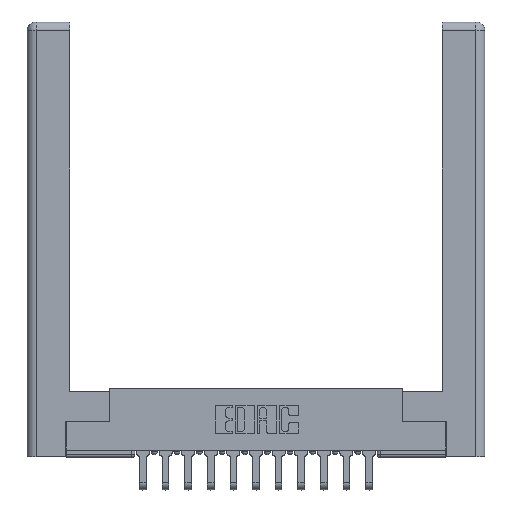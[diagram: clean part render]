
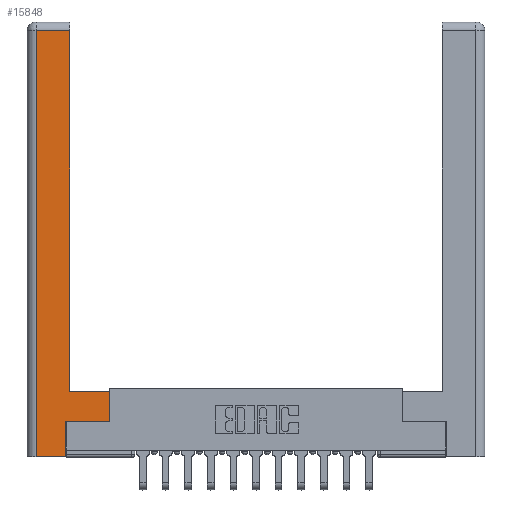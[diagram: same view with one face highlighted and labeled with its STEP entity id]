
A CAD part, top view. The second image highlights one B-rep face of the part: STEP entity #15848.
In plain terms, the highlighted planar face has unit normal (0, 0, 1).
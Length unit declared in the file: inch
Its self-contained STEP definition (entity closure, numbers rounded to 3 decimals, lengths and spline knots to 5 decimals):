
#21 = CARTESIAN_POINT ( 'NONE',  ( 0.265, 0.245, 0. ) ) ;
#48 = EDGE_CURVE ( 'NONE', #10854, #13648, #4577, .T. ) ;
#831 = VECTOR ( 'NONE', #4673, 39.37008 ) ;
#1161 = LINE ( 'NONE', #12009, #4280 ) ;
#1255 = CARTESIAN_POINT ( 'NONE',  ( 0.565, 0.45, 0. ) ) ;
#1319 = LINE ( 'NONE', #5548, #17010 ) ;
#1458 = LINE ( 'NONE', #21, #15605 ) ;
#1592 = VERTEX_POINT ( 'NONE', #5291 ) ;
#2045 = EDGE_CURVE ( 'NONE', #11021, #8924, #1319, .T. ) ;
#2308 = ORIENTED_EDGE ( 'NONE', *, *, #14729, .T. ) ;
#2418 = LINE ( 'NONE', #1255, #9904 ) ;
#2434 = LINE ( 'NONE', #6468, #12891 ) ;
#2515 = ORIENTED_EDGE ( 'NONE', *, *, #10357, .T. ) ;
#2670 = PLANE ( 'NONE',  #14595 ) ;
#2804 = EDGE_LOOP ( 'NONE', ( #8056, #16427, #3141, #2308, #14080, #10887, #13653, #2515 ) ) ;
#3123 = VECTOR ( 'NONE', #15313, 39.37008 ) ;
#3141 = ORIENTED_EDGE ( 'NONE', *, *, #11366, .T. ) ;
#3636 = CARTESIAN_POINT ( 'NONE',  ( 0.265, 0.245, 0. ) ) ;
#3809 = EDGE_CURVE ( 'NONE', #8924, #10315, #2418, .T. ) ;
#3841 = DIRECTION ( 'NONE',  ( 0., 0., -1. ) ) ;
#4144 = DIRECTION ( 'NONE',  ( 0., 1., 0. ) ) ;
#4280 = VECTOR ( 'NONE', #10565, 39.37008 ) ;
#4577 = LINE ( 'NONE', #15511, #831 ) ;
#4673 = DIRECTION ( 'NONE',  ( 0., 1., 0. ) ) ;
#4725 = EDGE_CURVE ( 'NONE', #11416, #11021, #1458, .T. ) ;
#5261 = CARTESIAN_POINT ( 'NONE',  ( 0.0615, 2.94, 0. ) ) ;
#5291 = CARTESIAN_POINT ( 'NONE',  ( 0.0615, 2.94, 0. ) ) ;
#5367 = VERTEX_POINT ( 'NONE', #11301 ) ;
#5545 = CARTESIAN_POINT ( 'NONE',  ( 0.565, 0.245, 0. ) ) ;
#5548 = CARTESIAN_POINT ( 'NONE',  ( 0.565, 0.245, 0. ) ) ;
#6095 = CARTESIAN_POINT ( 'NONE',  ( 0.565, 0.45, 0. ) ) ;
#6468 = CARTESIAN_POINT ( 'NONE',  ( 0.0615, 0., 0. ) ) ;
#6781 = DIRECTION ( 'NONE',  ( -1., 0., 0. ) ) ;
#8056 = ORIENTED_EDGE ( 'NONE', *, *, #48, .T. ) ;
#8129 = LINE ( 'NONE', #5261, #11469 ) ;
#8924 = VERTEX_POINT ( 'NONE', #5545 ) ;
#9904 = VECTOR ( 'NONE', #16128, 39.37008 ) ;
#10315 = VERTEX_POINT ( 'NONE', #6095 ) ;
#10357 = EDGE_CURVE ( 'NONE', #10315, #10854, #12900, .T. ) ;
#10565 = DIRECTION ( 'NONE',  ( 1., 0., 0. ) ) ;
#10774 = CARTESIAN_POINT ( 'NONE',  ( 0.265, 0., 0. ) ) ;
#10854 = VERTEX_POINT ( 'NONE', #16833 ) ;
#10887 = ORIENTED_EDGE ( 'NONE', *, *, #2045, .T. ) ;
#11021 = VERTEX_POINT ( 'NONE', #3636 ) ;
#11117 = EDGE_CURVE ( 'NONE', #13648, #1592, #8129, .T. ) ;
#11301 = CARTESIAN_POINT ( 'NONE',  ( 0.0615, 0., 0. ) ) ;
#11366 = EDGE_CURVE ( 'NONE', #1592, #5367, #2434, .T. ) ;
#11416 = VERTEX_POINT ( 'NONE', #10774 ) ;
#11469 = VECTOR ( 'NONE', #6781, 39.37008 ) ;
#11943 = DIRECTION ( 'NONE',  ( 0., -1., 0. ) ) ;
#12009 = CARTESIAN_POINT ( 'NONE',  ( 0.265, 0., 0. ) ) ;
#12180 = CARTESIAN_POINT ( 'NONE',  ( 0., 0., 0. ) ) ;
#12362 = FACE_OUTER_BOUND ( 'NONE', #2804, .T. ) ;
#12891 = VECTOR ( 'NONE', #11943, 39.37008 ) ;
#12900 = LINE ( 'NONE', #14151, #3123 ) ;
#13648 = VERTEX_POINT ( 'NONE', #17447 ) ;
#13653 = ORIENTED_EDGE ( 'NONE', *, *, #3809, .T. ) ;
#14080 = ORIENTED_EDGE ( 'NONE', *, *, #4725, .T. ) ;
#14151 = CARTESIAN_POINT ( 'NONE',  ( 0.295, 0.45, 0. ) ) ;
#14595 = AXIS2_PLACEMENT_3D ( 'NONE', #12180, #3841, #17548 ) ;
#14729 = EDGE_CURVE ( 'NONE', #5367, #11416, #1161, .T. ) ;
#15313 = DIRECTION ( 'NONE',  ( -1., 0., 0. ) ) ;
#15511 = CARTESIAN_POINT ( 'NONE',  ( 0.295, 3., 0. ) ) ;
#15605 = VECTOR ( 'NONE', #4144, 39.37008 ) ;
#15848 = ADVANCED_FACE ( 'NONE', ( #12362 ), #2670, .F. ) ;
#16128 = DIRECTION ( 'NONE',  ( 0., 1., 0. ) ) ;
#16374 = DIRECTION ( 'NONE',  ( 1., 0., 0. ) ) ;
#16427 = ORIENTED_EDGE ( 'NONE', *, *, #11117, .T. ) ;
#16833 = CARTESIAN_POINT ( 'NONE',  ( 0.295, 0.45, 0. ) ) ;
#17010 = VECTOR ( 'NONE', #16374, 39.37008 ) ;
#17447 = CARTESIAN_POINT ( 'NONE',  ( 0.295, 2.94, 0. ) ) ;
#17548 = DIRECTION ( 'NONE',  ( -1., 0., 0. ) ) ;
